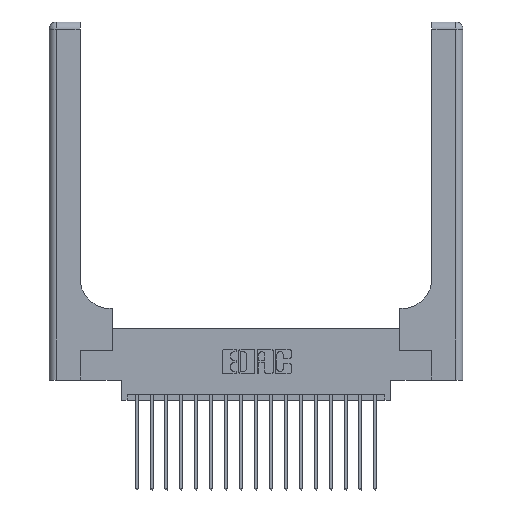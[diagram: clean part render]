
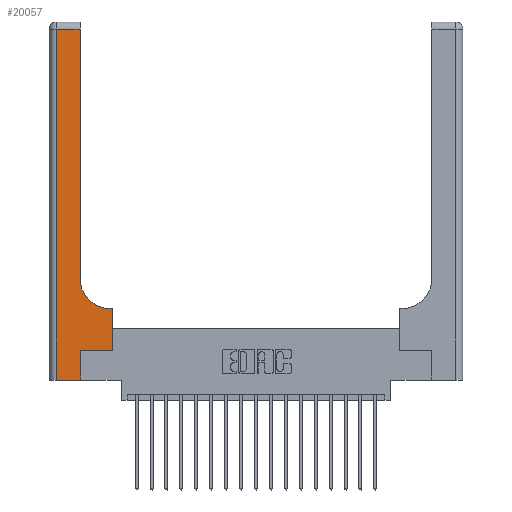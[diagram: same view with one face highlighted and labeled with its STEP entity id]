
A CAD part, top view. The second image highlights one B-rep face of the part: STEP entity #20057.
In plain terms, the highlighted planar face has unit normal (0, 0, 1).
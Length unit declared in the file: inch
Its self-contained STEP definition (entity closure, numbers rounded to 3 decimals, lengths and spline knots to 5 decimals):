
#321 = DIRECTION ( 'NONE',  ( 0., 0., -1. ) ) ;
#605 = EDGE_LOOP ( 'NONE', ( #1999, #11138, #8614, #7789, #8262, #8055, #9338, #8329, #1584 ) ) ;
#1285 = DIRECTION ( 'NONE',  ( 0., -1., 0. ) ) ;
#1306 = CARTESIAN_POINT ( 'NONE',  ( 0.26, 3., 0.37 ) ) ;
#1584 = ORIENTED_EDGE ( 'NONE', *, *, #14344, .T. ) ;
#1999 = ORIENTED_EDGE ( 'NONE', *, *, #4872, .T. ) ;
#2079 = CARTESIAN_POINT ( 'NONE',  ( 0.265, 0.25, 0.37 ) ) ;
#2150 = VECTOR ( 'NONE', #19309, 39.37008 ) ;
#2342 = VERTEX_POINT ( 'NONE', #15760 ) ;
#2456 = DIRECTION ( 'NONE',  ( 0., 1., 0. ) ) ;
#2469 = LINE ( 'NONE', #10163, #17379 ) ;
#2738 = PLANE ( 'NONE',  #16880 ) ;
#3771 = EDGE_CURVE ( 'NONE', #16254, #7914, #4966, .T. ) ;
#4159 = LINE ( 'NONE', #8780, #14252 ) ;
#4347 = LINE ( 'NONE', #5885, #12567 ) ;
#4468 = DIRECTION ( 'NONE',  ( 0., 1., 0. ) ) ;
#4513 = VERTEX_POINT ( 'NONE', #9618 ) ;
#4573 = DIRECTION ( 'NONE',  ( -1., 0., 0. ) ) ;
#4872 = EDGE_CURVE ( 'NONE', #16489, #14213, #6004, .T. ) ;
#4966 = LINE ( 'NONE', #14297, #11224 ) ;
#5885 = CARTESIAN_POINT ( 'NONE',  ( 0.06, 3., 0.37 ) ) ;
#5915 = CARTESIAN_POINT ( 'NONE',  ( 0., 3., 0.37 ) ) ;
#6004 = LINE ( 'NONE', #1306, #11350 ) ;
#6262 = CARTESIAN_POINT ( 'NONE',  ( 0.51, 0.85, 0.37 ) ) ;
#6357 = EDGE_CURVE ( 'NONE', #4513, #2342, #16051, .T. ) ;
#6439 = VERTEX_POINT ( 'NONE', #19407 ) ;
#6529 = VERTEX_POINT ( 'NONE', #15515 ) ;
#7208 = CARTESIAN_POINT ( 'NONE',  ( 0.528, 0.25, 0.37 ) ) ;
#7265 = CARTESIAN_POINT ( 'NONE',  ( 0.51, 0.6, 0.37 ) ) ;
#7789 = ORIENTED_EDGE ( 'NONE', *, *, #6357, .T. ) ;
#7839 = DIRECTION ( 'NONE',  ( 1., 0., 0. ) ) ;
#7914 = VERTEX_POINT ( 'NONE', #10587 ) ;
#8055 = ORIENTED_EDGE ( 'NONE', *, *, #3771, .T. ) ;
#8262 = ORIENTED_EDGE ( 'NONE', *, *, #16796, .T. ) ;
#8267 = CARTESIAN_POINT ( 'NONE',  ( 0., 0., 0.37 ) ) ;
#8329 = ORIENTED_EDGE ( 'NONE', *, *, #17386, .T. ) ;
#8614 = ORIENTED_EDGE ( 'NONE', *, *, #14916, .T. ) ;
#8615 = LINE ( 'NONE', #11597, #18479 ) ;
#8735 = DIRECTION ( 'NONE',  ( -1., 0., 0. ) ) ;
#8780 = CARTESIAN_POINT ( 'NONE',  ( 0.26, 0.6, 0.37 ) ) ;
#8993 = DIRECTION ( 'NONE',  ( 0., 0., -1. ) ) ;
#9251 = CARTESIAN_POINT ( 'NONE',  ( 0.26, 0.85, 0.37 ) ) ;
#9338 = ORIENTED_EDGE ( 'NONE', *, *, #16317, .T. ) ;
#9618 = CARTESIAN_POINT ( 'NONE',  ( 0.06, 0., 0.37 ) ) ;
#9752 = VERTEX_POINT ( 'NONE', #7265 ) ;
#10163 = CARTESIAN_POINT ( 'NONE',  ( 0., 2.94, 0.37 ) ) ;
#10536 = EDGE_CURVE ( 'NONE', #14213, #6439, #2469, .T. ) ;
#10587 = CARTESIAN_POINT ( 'NONE',  ( 0.528, 0.25, 0.37 ) ) ;
#11138 = ORIENTED_EDGE ( 'NONE', *, *, #10536, .T. ) ;
#11224 = VECTOR ( 'NONE', #7839, 39.37008 ) ;
#11350 = VECTOR ( 'NONE', #4468, 39.37008 ) ;
#11597 = CARTESIAN_POINT ( 'NONE',  ( 0.265, 0., 0.37 ) ) ;
#12221 = AXIS2_PLACEMENT_3D ( 'NONE', #6262, #321, #12738 ) ;
#12567 = VECTOR ( 'NONE', #1285, 39.37008 ) ;
#12738 = DIRECTION ( 'NONE',  ( 1., 0., 0. ) ) ;
#13248 = VECTOR ( 'NONE', #18162, 39.37008 ) ;
#14213 = VERTEX_POINT ( 'NONE', #19185 ) ;
#14252 = VECTOR ( 'NONE', #16661, 39.37008 ) ;
#14297 = CARTESIAN_POINT ( 'NONE',  ( 0.265, 0.25, 0.37 ) ) ;
#14344 = EDGE_CURVE ( 'NONE', #9752, #16489, #20037, .T. ) ;
#14916 = EDGE_CURVE ( 'NONE', #6439, #4513, #4347, .T. ) ;
#15515 = CARTESIAN_POINT ( 'NONE',  ( 0.528, 0.6, 0.37 ) ) ;
#15760 = CARTESIAN_POINT ( 'NONE',  ( 0.265, 0., 0.37 ) ) ;
#16051 = LINE ( 'NONE', #8267, #2150 ) ;
#16254 = VERTEX_POINT ( 'NONE', #2079 ) ;
#16317 = EDGE_CURVE ( 'NONE', #7914, #6529, #17956, .T. ) ;
#16489 = VERTEX_POINT ( 'NONE', #9251 ) ;
#16661 = DIRECTION ( 'NONE',  ( -1., 0., 0. ) ) ;
#16796 = EDGE_CURVE ( 'NONE', #2342, #16254, #8615, .T. ) ;
#16880 = AXIS2_PLACEMENT_3D ( 'NONE', #5915, #8993, #4573 ) ;
#17379 = VECTOR ( 'NONE', #8735, 39.37008 ) ;
#17386 = EDGE_CURVE ( 'NONE', #6529, #9752, #4159, .T. ) ;
#17956 = LINE ( 'NONE', #7208, #13248 ) ;
#18162 = DIRECTION ( 'NONE',  ( 0., 1., 0. ) ) ;
#18479 = VECTOR ( 'NONE', #2456, 39.37008 ) ;
#19185 = CARTESIAN_POINT ( 'NONE',  ( 0.26, 2.94, 0.37 ) ) ;
#19309 = DIRECTION ( 'NONE',  ( 1., 0., 0. ) ) ;
#19407 = CARTESIAN_POINT ( 'NONE',  ( 0.06, 2.94, 0.37 ) ) ;
#19934 = FACE_OUTER_BOUND ( 'NONE', #605, .T. ) ;
#20037 = CIRCLE ( 'NONE', #12221, 0.25 ) ;
#20057 = ADVANCED_FACE ( 'NONE', ( #19934 ), #2738, .F. ) ;
